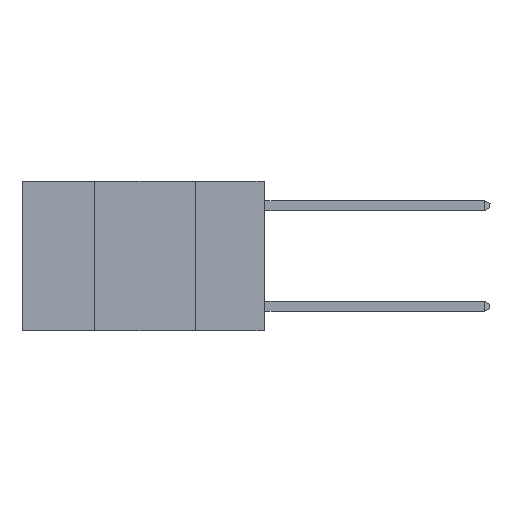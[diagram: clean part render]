
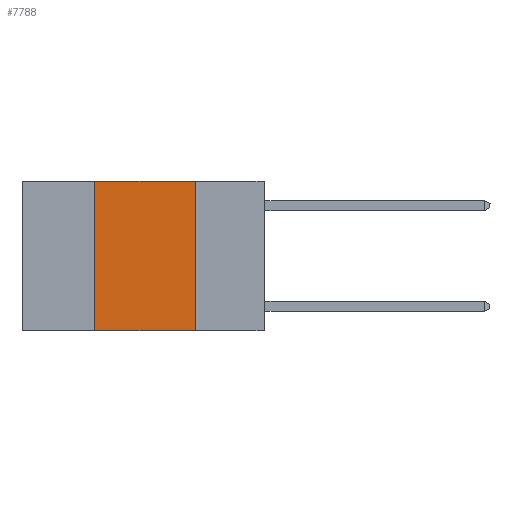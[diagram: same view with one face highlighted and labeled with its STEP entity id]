
A CAD part, left-side view. The second image highlights one B-rep face of the part: STEP entity #7788.
In plain terms, the highlighted planar face has unit normal (-1, 0, 0).
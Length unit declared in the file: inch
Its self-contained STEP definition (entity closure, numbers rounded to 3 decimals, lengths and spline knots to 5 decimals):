
#511 = CARTESIAN_POINT ( 'NONE',  ( 0., 0.17, -0.37 ) ) ;
#771 = DIRECTION ( 'NONE',  ( 0., -1., 0. ) ) ;
#986 = VECTOR ( 'NONE', #4359, 39.37008 ) ;
#1355 = VECTOR ( 'NONE', #7335, 39.37008 ) ;
#1415 = EDGE_CURVE ( 'NONE', #2659, #3950, #2083, .T. ) ;
#1427 = CARTESIAN_POINT ( 'NONE',  ( 0., 0.6, -0.37 ) ) ;
#2078 = PLANE ( 'NONE',  #2138 ) ;
#2083 = LINE ( 'NONE', #4437, #1355 ) ;
#2138 = AXIS2_PLACEMENT_3D ( 'NONE', #4987, #7214, #5028 ) ;
#2243 = CARTESIAN_POINT ( 'NONE',  ( 0., 0.17, 0. ) ) ;
#2659 = VERTEX_POINT ( 'NONE', #5128 ) ;
#2865 = LINE ( 'NONE', #6565, #3058 ) ;
#2982 = ORIENTED_EDGE ( 'NONE', *, *, #8173, .F. ) ;
#3058 = VECTOR ( 'NONE', #7810, 39.37008 ) ;
#3825 = VECTOR ( 'NONE', #771, 39.37008 ) ;
#3950 = VERTEX_POINT ( 'NONE', #4050 ) ;
#4050 = CARTESIAN_POINT ( 'NONE',  ( 0., 0.42, 0. ) ) ;
#4359 = DIRECTION ( 'NONE',  ( 0., -1., 0. ) ) ;
#4420 = LINE ( 'NONE', #7320, #3825 ) ;
#4437 = CARTESIAN_POINT ( 'NONE',  ( 0., 0.42, 0. ) ) ;
#4549 = ORIENTED_EDGE ( 'NONE', *, *, #5567, .F. ) ;
#4987 = CARTESIAN_POINT ( 'NONE',  ( 0., 0.6, 0. ) ) ;
#4989 = ORIENTED_EDGE ( 'NONE', *, *, #1415, .F. ) ;
#5028 = DIRECTION ( 'NONE',  ( 0., 0., -1. ) ) ;
#5128 = CARTESIAN_POINT ( 'NONE',  ( 0., 0.42, -0.37 ) ) ;
#5567 = EDGE_CURVE ( 'NONE', #3950, #9414, #4420, .T. ) ;
#6249 = VERTEX_POINT ( 'NONE', #511 ) ;
#6528 = FACE_OUTER_BOUND ( 'NONE', #8157, .T. ) ;
#6565 = CARTESIAN_POINT ( 'NONE',  ( 0., 0.17, 0. ) ) ;
#7214 = DIRECTION ( 'NONE',  ( 1., 0., 0. ) ) ;
#7320 = CARTESIAN_POINT ( 'NONE',  ( 0., 0.6, 0. ) ) ;
#7335 = DIRECTION ( 'NONE',  ( 0., 0., 1. ) ) ;
#7411 = EDGE_CURVE ( 'NONE', #2659, #6249, #9411, .T. ) ;
#7788 = ADVANCED_FACE ( 'NONE', ( #6528 ), #2078, .F. ) ;
#7810 = DIRECTION ( 'NONE',  ( 0., 0., -1. ) ) ;
#8157 = EDGE_LOOP ( 'NONE', ( #2982, #4549, #4989, #8550 ) ) ;
#8173 = EDGE_CURVE ( 'NONE', #9414, #6249, #2865, .T. ) ;
#8550 = ORIENTED_EDGE ( 'NONE', *, *, #7411, .T. ) ;
#9411 = LINE ( 'NONE', #1427, #986 ) ;
#9414 = VERTEX_POINT ( 'NONE', #2243 ) ;
